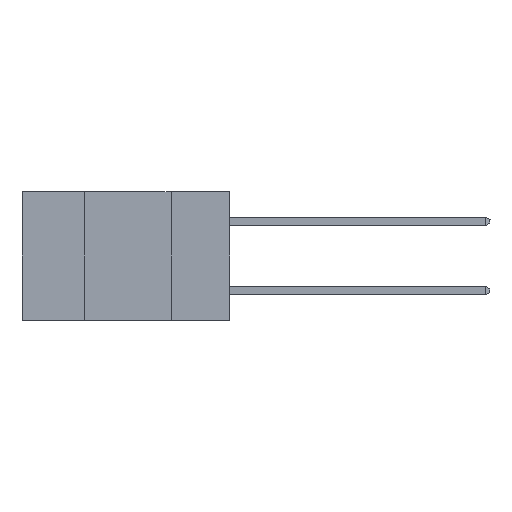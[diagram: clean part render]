
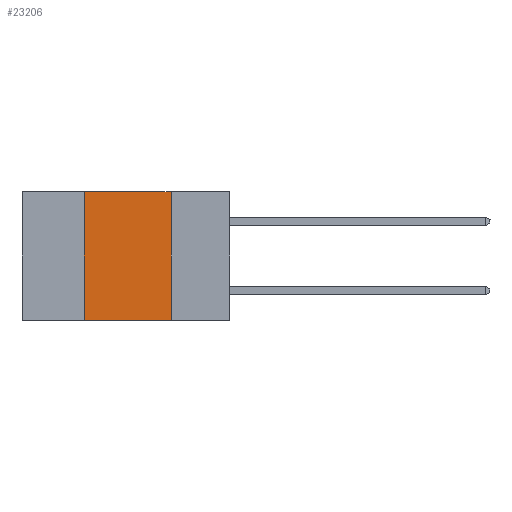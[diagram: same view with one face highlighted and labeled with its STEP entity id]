
A CAD part, left-side view. The second image highlights one B-rep face of the part: STEP entity #23206.
In plain terms, the highlighted planar face has unit normal (-1, 0, 0).
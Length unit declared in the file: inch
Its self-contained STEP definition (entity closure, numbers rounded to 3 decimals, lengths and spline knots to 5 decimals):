
#227 = DIRECTION ( 'NONE',  ( 0., -1., 0. ) ) ;
#1552 = FACE_OUTER_BOUND ( 'NONE', #26975, .T. ) ;
#1955 = LINE ( 'NONE', #27088, #17716 ) ;
#6059 = CARTESIAN_POINT ( 'NONE',  ( 0., 0.17, 0. ) ) ;
#6549 = CARTESIAN_POINT ( 'NONE',  ( 0., 0.17, -0.37 ) ) ;
#7194 = EDGE_CURVE ( 'NONE', #9690, #9404, #30299, .T. ) ;
#9108 = PLANE ( 'NONE',  #28306 ) ;
#9404 = VERTEX_POINT ( 'NONE', #16120 ) ;
#9690 = VERTEX_POINT ( 'NONE', #28949 ) ;
#10037 = CARTESIAN_POINT ( 'NONE',  ( 0., 0.6, 0. ) ) ;
#10588 = EDGE_CURVE ( 'NONE', #28878, #30631, #29613, .T. ) ;
#10869 = ORIENTED_EDGE ( 'NONE', *, *, #29518, .F. ) ;
#11565 = DIRECTION ( 'NONE',  ( 0., 0., -1. ) ) ;
#12989 = ORIENTED_EDGE ( 'NONE', *, *, #10588, .T. ) ;
#14891 = DIRECTION ( 'NONE',  ( 0., -1., 0. ) ) ;
#16120 = CARTESIAN_POINT ( 'NONE',  ( 0., 0.17, 0. ) ) ;
#16239 = VECTOR ( 'NONE', #227, 39.37008 ) ;
#16674 = DIRECTION ( 'NONE',  ( 1., 0., 0. ) ) ;
#17007 = LINE ( 'NONE', #6059, #31552 ) ;
#17217 = CARTESIAN_POINT ( 'NONE',  ( 0., 0.42, -0.37 ) ) ;
#17716 = VECTOR ( 'NONE', #19772, 39.37008 ) ;
#19772 = DIRECTION ( 'NONE',  ( 0., 0., 1. ) ) ;
#22468 = EDGE_CURVE ( 'NONE', #9404, #30631, #17007, .T. ) ;
#23206 = ADVANCED_FACE ( 'NONE', ( #1552 ), #9108, .F. ) ;
#23270 = VECTOR ( 'NONE', #14891, 39.37008 ) ;
#26970 = ORIENTED_EDGE ( 'NONE', *, *, #7194, .F. ) ;
#26975 = EDGE_LOOP ( 'NONE', ( #29710, #26970, #10869, #12989 ) ) ;
#27088 = CARTESIAN_POINT ( 'NONE',  ( 0., 0.42, 0. ) ) ;
#28082 = CARTESIAN_POINT ( 'NONE',  ( 0., 0.6, -0.37 ) ) ;
#28306 = AXIS2_PLACEMENT_3D ( 'NONE', #29415, #16674, #29528 ) ;
#28878 = VERTEX_POINT ( 'NONE', #17217 ) ;
#28949 = CARTESIAN_POINT ( 'NONE',  ( 0., 0.42, 0. ) ) ;
#29415 = CARTESIAN_POINT ( 'NONE',  ( 0., 0.6, 0. ) ) ;
#29518 = EDGE_CURVE ( 'NONE', #28878, #9690, #1955, .T. ) ;
#29528 = DIRECTION ( 'NONE',  ( 0., 0., -1. ) ) ;
#29613 = LINE ( 'NONE', #28082, #16239 ) ;
#29710 = ORIENTED_EDGE ( 'NONE', *, *, #22468, .F. ) ;
#30299 = LINE ( 'NONE', #10037, #23270 ) ;
#30631 = VERTEX_POINT ( 'NONE', #6549 ) ;
#31552 = VECTOR ( 'NONE', #11565, 39.37008 ) ;
